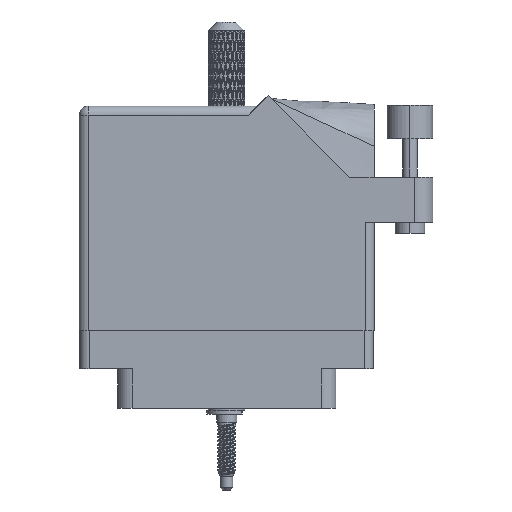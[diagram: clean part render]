
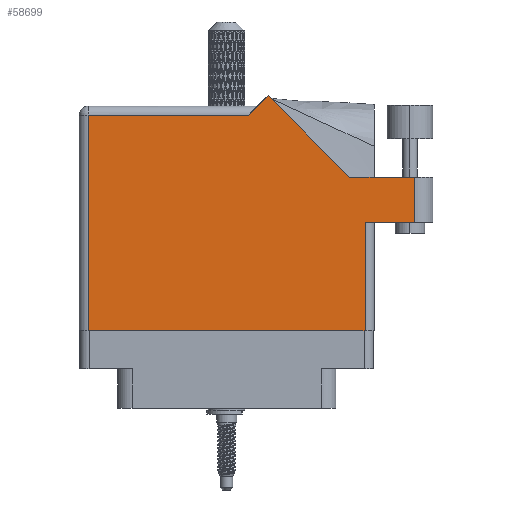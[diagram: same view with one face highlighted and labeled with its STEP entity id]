
A CAD part, front view. The second image highlights one B-rep face of the part: STEP entity #58699.
In plain terms, the highlighted face is planar.
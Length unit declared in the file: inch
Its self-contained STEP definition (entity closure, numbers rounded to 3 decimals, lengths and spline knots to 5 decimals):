
#930 = VERTEX_POINT ( 'NONE', #84050 ) ;
#1241 = DIRECTION ( 'NONE',  ( -1., 0., 0. ) ) ;
#1568 = CARTESIAN_POINT ( 'NONE',  ( 2.285, 0.737, 0. ) ) ;
#4310 = LINE ( 'NONE', #11750, #69670 ) ;
#4557 = ORIENTED_EDGE ( 'NONE', *, *, #53755, .T. ) ;
#5246 = ORIENTED_EDGE ( 'NONE', *, *, #49493, .T. ) ;
#6487 = PLANE ( 'NONE',  #11698 ) ;
#7787 = DIRECTION ( 'NONE',  ( -1., 0., 0. ) ) ;
#10282 = VERTEX_POINT ( 'NONE', #96120 ) ;
#10471 = LINE ( 'NONE', #99968, #31738 ) ;
#11698 = AXIS2_PLACEMENT_3D ( 'NONE', #45740, #39917, #13398 ) ;
#11750 = CARTESIAN_POINT ( 'NONE',  ( 2.01, 0.737, 0. ) ) ;
#12035 = VERTEX_POINT ( 'NONE', #21864 ) ;
#13398 = DIRECTION ( 'NONE',  ( -1., 0., 0. ) ) ;
#16268 = CARTESIAN_POINT ( 'NONE',  ( 2.41, 1.044, 0. ) ) ;
#16985 = VECTOR ( 'NONE', #72069, 39.37008 ) ;
#21864 = CARTESIAN_POINT ( 'NONE',  ( 1.28771, 1.60071, 0. ) ) ;
#22160 = VECTOR ( 'NONE', #87876, 39.37008 ) ;
#23439 = CARTESIAN_POINT ( 'NONE',  ( 0.062, 0., 0. ) ) ;
#25451 = ORIENTED_EDGE ( 'NONE', *, *, #62678, .T. ) ;
#28557 = VECTOR ( 'NONE', #56857, 39.37008 ) ;
#29278 = VERTEX_POINT ( 'NONE', #37611 ) ;
#29662 = CARTESIAN_POINT ( 'NONE',  ( 1.84442, 1.044, 0. ) ) ;
#29857 = FACE_OUTER_BOUND ( 'NONE', #32980, .T. ) ;
#31738 = VECTOR ( 'NONE', #32935, 39.37008 ) ;
#31740 = CARTESIAN_POINT ( 'NONE',  ( 1.217, 1.53, 0. ) ) ;
#32935 = DIRECTION ( 'NONE',  ( 0., 1., 0. ) ) ;
#32980 = EDGE_LOOP ( 'NONE', ( #50491, #58141, #56562, #5246, #25451, #68803, #94031, #4557, #101682 ) ) ;
#37611 = CARTESIAN_POINT ( 'NONE',  ( 0.062, 0., 0. ) ) ;
#37641 = DIRECTION ( 'NONE',  ( -0.707, 0.707, 0. ) ) ;
#39917 = DIRECTION ( 'NONE',  ( 0., 0., -1. ) ) ;
#40545 = EDGE_CURVE ( 'NONE', #10282, #48333, #10471, .T. ) ;
#41585 = LINE ( 'NONE', #73870, #62846 ) ;
#45740 = CARTESIAN_POINT ( 'NONE',  ( 0., 1.53, 0. ) ) ;
#48333 = VERTEX_POINT ( 'NONE', #60921 ) ;
#49493 = EDGE_CURVE ( 'NONE', #66798, #12035, #78404, .T. ) ;
#50491 = ORIENTED_EDGE ( 'NONE', *, *, #56642, .T. ) ;
#51274 = EDGE_CURVE ( 'NONE', #100319, #930, #41585, .T. ) ;
#53755 = EDGE_CURVE ( 'NONE', #29278, #10282, #72597, .T. ) ;
#56562 = ORIENTED_EDGE ( 'NONE', *, *, #64593, .T. ) ;
#56642 = EDGE_CURVE ( 'NONE', #48333, #96124, #4310, .T. ) ;
#56857 = DIRECTION ( 'NONE',  ( 0., -1., 0. ) ) ;
#58043 = CARTESIAN_POINT ( 'NONE',  ( 1.155, 1.468, 0. ) ) ;
#58141 = ORIENTED_EDGE ( 'NONE', *, *, #63538, .T. ) ;
#58699 = ADVANCED_FACE ( 'NONE', ( #29857 ), #6487, .F. ) ;
#60387 = VERTEX_POINT ( 'NONE', #75081 ) ;
#60801 = CARTESIAN_POINT ( 'NONE',  ( 1.84442, 1.044, 0. ) ) ;
#60921 = CARTESIAN_POINT ( 'NONE',  ( 1.948, 0.737, 0. ) ) ;
#61616 = DIRECTION ( 'NONE',  ( 1., 0., 0. ) ) ;
#62678 = EDGE_CURVE ( 'NONE', #12035, #100319, #88395, .T. ) ;
#62846 = VECTOR ( 'NONE', #1241, 39.37008 ) ;
#63538 = EDGE_CURVE ( 'NONE', #96124, #60387, #103758, .T. ) ;
#63568 = DIRECTION ( 'NONE',  ( 0., 1., 0. ) ) ;
#64593 = EDGE_CURVE ( 'NONE', #60387, #66798, #74025, .T. ) ;
#64650 = VECTOR ( 'NONE', #7787, 39.37008 ) ;
#66798 = VERTEX_POINT ( 'NONE', #60801 ) ;
#68803 = ORIENTED_EDGE ( 'NONE', *, *, #51274, .T. ) ;
#69605 = VECTOR ( 'NONE', #63568, 39.37008 ) ;
#69670 = VECTOR ( 'NONE', #61616, 39.37008 ) ;
#71482 = CARTESIAN_POINT ( 'NONE',  ( 2.285, 1.044, 0. ) ) ;
#71559 = CARTESIAN_POINT ( 'NONE',  ( 0., 0., 0. ) ) ;
#72069 = DIRECTION ( 'NONE',  ( 1., 0., 0. ) ) ;
#72597 = LINE ( 'NONE', #71559, #16985 ) ;
#73870 = CARTESIAN_POINT ( 'NONE',  ( 0., 1.468, 0. ) ) ;
#73878 = EDGE_CURVE ( 'NONE', #930, #29278, #79115, .T. ) ;
#74025 = LINE ( 'NONE', #16268, #64650 ) ;
#75081 = CARTESIAN_POINT ( 'NONE',  ( 2.285, 1.044, 0. ) ) ;
#78404 = LINE ( 'NONE', #29662, #102380 ) ;
#79115 = LINE ( 'NONE', #23439, #28557 ) ;
#84050 = CARTESIAN_POINT ( 'NONE',  ( 0.062, 1.468, 0. ) ) ;
#87876 = DIRECTION ( 'NONE',  ( -0.707, -0.707, 0. ) ) ;
#88395 = LINE ( 'NONE', #31740, #22160 ) ;
#94031 = ORIENTED_EDGE ( 'NONE', *, *, #73878, .T. ) ;
#96120 = CARTESIAN_POINT ( 'NONE',  ( 1.948, 0., 0. ) ) ;
#96124 = VERTEX_POINT ( 'NONE', #1568 ) ;
#99968 = CARTESIAN_POINT ( 'NONE',  ( 1.948, 0.737, 0. ) ) ;
#100319 = VERTEX_POINT ( 'NONE', #58043 ) ;
#101682 = ORIENTED_EDGE ( 'NONE', *, *, #40545, .T. ) ;
#102380 = VECTOR ( 'NONE', #37641, 39.37008 ) ;
#103758 = LINE ( 'NONE', #71482, #69605 ) ;
